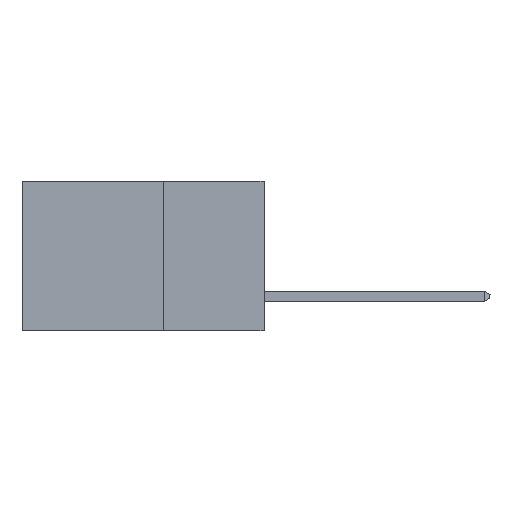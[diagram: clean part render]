
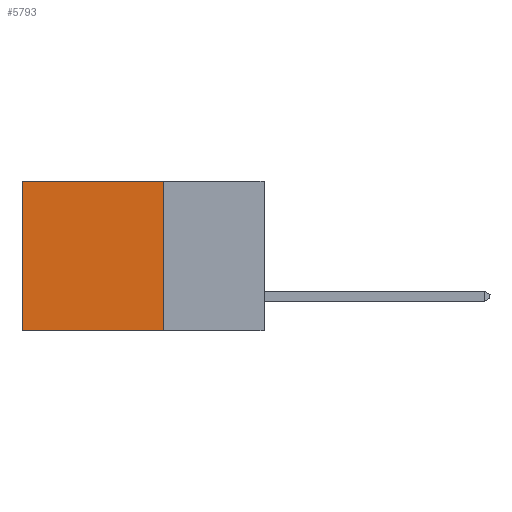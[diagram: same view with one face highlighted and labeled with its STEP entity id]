
A CAD part, left-side view. The second image highlights one B-rep face of the part: STEP entity #5793.
In plain terms, the highlighted planar face has unit normal (-1, 0, 0).
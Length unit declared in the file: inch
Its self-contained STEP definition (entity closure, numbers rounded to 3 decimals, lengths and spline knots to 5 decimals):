
#39 = CARTESIAN_POINT ( 'NONE',  ( 0.2615, 0.25, -0.37 ) ) ;
#524 = EDGE_CURVE ( 'NONE', #10362, #7973, #2938, .T. ) ;
#635 = DIRECTION ( 'NONE',  ( 0., 1., 0. ) ) ;
#781 = DIRECTION ( 'NONE',  ( 0., 0., -1. ) ) ;
#1056 = PLANE ( 'NONE',  #6913 ) ;
#1768 = EDGE_CURVE ( 'NONE', #7058, #10362, #4851, .T. ) ;
#2147 = CARTESIAN_POINT ( 'NONE',  ( 0.2615, 0.25, 0. ) ) ;
#2419 = ORIENTED_EDGE ( 'NONE', *, *, #9925, .F. ) ;
#2422 = DIRECTION ( 'NONE',  ( 0., 1., 0. ) ) ;
#2760 = CARTESIAN_POINT ( 'NONE',  ( 0.2615, 0.25, 0. ) ) ;
#2763 = CARTESIAN_POINT ( 'NONE',  ( 0.2615, 0.6, 0. ) ) ;
#2873 = DIRECTION ( 'NONE',  ( 0., 0., -1. ) ) ;
#2938 = LINE ( 'NONE', #9317, #11362 ) ;
#3042 = FACE_OUTER_BOUND ( 'NONE', #11499, .T. ) ;
#3607 = VECTOR ( 'NONE', #635, 39.37008 ) ;
#4832 = ORIENTED_EDGE ( 'NONE', *, *, #8491, .F. ) ;
#4851 = LINE ( 'NONE', #2760, #3607 ) ;
#4896 = CARTESIAN_POINT ( 'NONE',  ( 0.2615, 0.6, -0.37 ) ) ;
#5397 = VERTEX_POINT ( 'NONE', #10364 ) ;
#5793 = ADVANCED_FACE ( 'NONE', ( #3042 ), #1056, .F. ) ;
#5945 = DIRECTION ( 'NONE',  ( 1., 0., 0. ) ) ;
#6492 = VECTOR ( 'NONE', #2422, 39.37008 ) ;
#6913 = AXIS2_PLACEMENT_3D ( 'NONE', #39, #5945, #781 ) ;
#7058 = VERTEX_POINT ( 'NONE', #2147 ) ;
#7119 = DIRECTION ( 'NONE',  ( 0., 0., -1. ) ) ;
#7168 = ORIENTED_EDGE ( 'NONE', *, *, #524, .T. ) ;
#7973 = VERTEX_POINT ( 'NONE', #4896 ) ;
#8491 = EDGE_CURVE ( 'NONE', #5397, #7973, #9742, .T. ) ;
#9317 = CARTESIAN_POINT ( 'NONE',  ( 0.2615, 0.6, -0.37 ) ) ;
#9742 = LINE ( 'NONE', #12710, #6492 ) ;
#9925 = EDGE_CURVE ( 'NONE', #7058, #5397, #13335, .T. ) ;
#10362 = VERTEX_POINT ( 'NONE', #2763 ) ;
#10364 = CARTESIAN_POINT ( 'NONE',  ( 0.2615, 0.25, -0.37 ) ) ;
#11362 = VECTOR ( 'NONE', #2873, 39.37008 ) ;
#11499 = EDGE_LOOP ( 'NONE', ( #7168, #4832, #2419, #12313 ) ) ;
#11706 = VECTOR ( 'NONE', #7119, 39.37008 ) ;
#12313 = ORIENTED_EDGE ( 'NONE', *, *, #1768, .T. ) ;
#12710 = CARTESIAN_POINT ( 'NONE',  ( 0.2615, 0.25, -0.37 ) ) ;
#13206 = CARTESIAN_POINT ( 'NONE',  ( 0.2615, 0.25, -0.37 ) ) ;
#13335 = LINE ( 'NONE', #13206, #11706 ) ;
